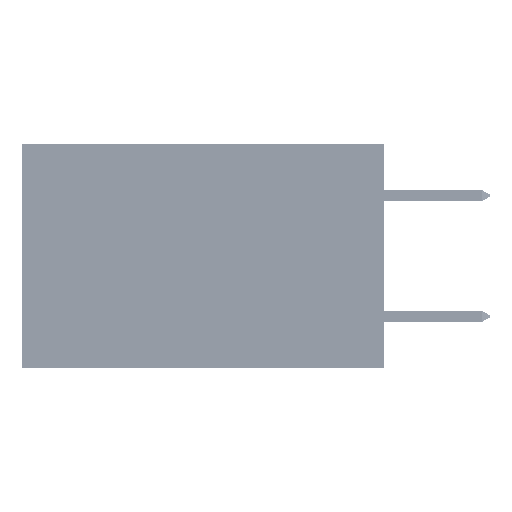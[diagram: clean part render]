
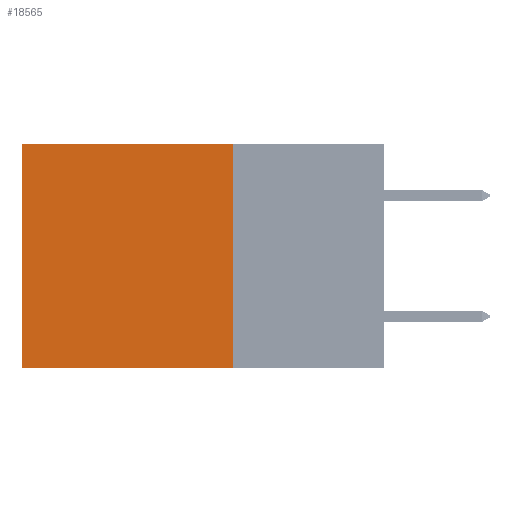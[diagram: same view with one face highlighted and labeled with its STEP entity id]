
A CAD part, left-side view. The second image highlights one B-rep face of the part: STEP entity #18565.
In plain terms, the highlighted planar face has unit normal (-1, 0, 0).
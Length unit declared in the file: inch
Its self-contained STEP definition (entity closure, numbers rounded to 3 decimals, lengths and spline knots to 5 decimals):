
#1019 = VERTEX_POINT ( 'NONE', #4017 ) ;
#3426 = VERTEX_POINT ( 'NONE', #46315 ) ;
#4017 = CARTESIAN_POINT ( 'NONE',  ( 0.2875, 0.25, 0. ) ) ;
#5020 = VERTEX_POINT ( 'NONE', #11695 ) ;
#5108 = VECTOR ( 'NONE', #30739, 39.37008 ) ;
#5878 = AXIS2_PLACEMENT_3D ( 'NONE', #30567, #18738, #46012 ) ;
#6152 = EDGE_CURVE ( 'NONE', #1019, #48255, #15363, .T. ) ;
#8535 = VECTOR ( 'NONE', #32025, 39.37008 ) ;
#11340 = DIRECTION ( 'NONE',  ( 0., 1., 0. ) ) ;
#11695 = CARTESIAN_POINT ( 'NONE',  ( 0.2875, 0.6, 0. ) ) ;
#11866 = CARTESIAN_POINT ( 'NONE',  ( 0.2875, 0.25, 0. ) ) ;
#11938 = ORIENTED_EDGE ( 'NONE', *, *, #23416, .F. ) ;
#12954 = CARTESIAN_POINT ( 'NONE',  ( 0.2875, 0.6, 0. ) ) ;
#15096 = FACE_OUTER_BOUND ( 'NONE', #18415, .T. ) ;
#15363 = LINE ( 'NONE', #11866, #5108 ) ;
#18415 = EDGE_LOOP ( 'NONE', ( #24068, #11938, #49820, #37079 ) ) ;
#18565 = ADVANCED_FACE ( 'NONE', ( #15096 ), #37292, .F. ) ;
#18738 = DIRECTION ( 'NONE',  ( 1., 0., 0. ) ) ;
#19431 = VECTOR ( 'NONE', #21724, 39.37008 ) ;
#19756 = CARTESIAN_POINT ( 'NONE',  ( 0.2875, 0.25, -0.37 ) ) ;
#21724 = DIRECTION ( 'NONE',  ( 0., 1., 0. ) ) ;
#23416 = EDGE_CURVE ( 'NONE', #48255, #3426, #47766, .T. ) ;
#24011 = EDGE_CURVE ( 'NONE', #5020, #3426, #45299, .T. ) ;
#24068 = ORIENTED_EDGE ( 'NONE', *, *, #24011, .T. ) ;
#28100 = EDGE_CURVE ( 'NONE', #1019, #5020, #37332, .T. ) ;
#30567 = CARTESIAN_POINT ( 'NONE',  ( 0.2875, 0.25, 0. ) ) ;
#30739 = DIRECTION ( 'NONE',  ( 0., 0., -1. ) ) ;
#32025 = DIRECTION ( 'NONE',  ( 0., 0., -1. ) ) ;
#37079 = ORIENTED_EDGE ( 'NONE', *, *, #28100, .T. ) ;
#37292 = PLANE ( 'NONE',  #5878 ) ;
#37332 = LINE ( 'NONE', #45830, #39157 ) ;
#39157 = VECTOR ( 'NONE', #11340, 39.37008 ) ;
#43991 = CARTESIAN_POINT ( 'NONE',  ( 0.2875, 0.25, -0.37 ) ) ;
#45299 = LINE ( 'NONE', #12954, #8535 ) ;
#45830 = CARTESIAN_POINT ( 'NONE',  ( 0.2875, 0.25, 0. ) ) ;
#46012 = DIRECTION ( 'NONE',  ( 0., 0., -1. ) ) ;
#46315 = CARTESIAN_POINT ( 'NONE',  ( 0.2875, 0.6, -0.37 ) ) ;
#47766 = LINE ( 'NONE', #43991, #19431 ) ;
#48255 = VERTEX_POINT ( 'NONE', #19756 ) ;
#49820 = ORIENTED_EDGE ( 'NONE', *, *, #6152, .F. ) ;
